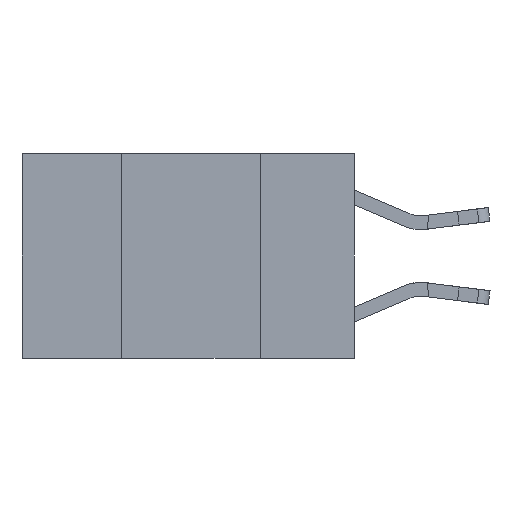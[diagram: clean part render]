
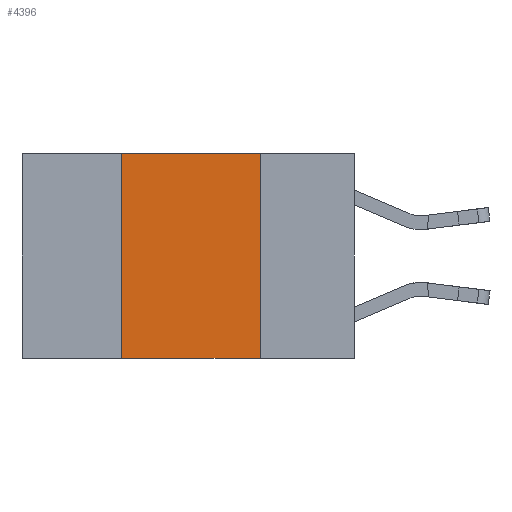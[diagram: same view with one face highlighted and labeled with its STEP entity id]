
A CAD part, left-side view. The second image highlights one B-rep face of the part: STEP entity #4396.
In plain terms, the highlighted planar face has unit normal (-1, 0, 0).
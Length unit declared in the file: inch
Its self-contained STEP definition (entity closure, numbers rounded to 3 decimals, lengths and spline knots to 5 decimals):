
#115 = CARTESIAN_POINT ( 'NONE',  ( 0., 0.42, 0. ) ) ;
#426 = VERTEX_POINT ( 'NONE', #19017 ) ;
#518 = LINE ( 'NONE', #115, #14392 ) ;
#2198 = CARTESIAN_POINT ( 'NONE',  ( 0., 0.42, -0.37 ) ) ;
#3190 = DIRECTION ( 'NONE',  ( 1., 0., 0. ) ) ;
#3238 = VECTOR ( 'NONE', #23253, 39.37008 ) ;
#3935 = ORIENTED_EDGE ( 'NONE', *, *, #14655, .F. ) ;
#4396 = ADVANCED_FACE ( 'NONE', ( #26177 ), #24254, .F. ) ;
#5618 = LINE ( 'NONE', #13851, #10953 ) ;
#5630 = CARTESIAN_POINT ( 'NONE',  ( 0., 0.17, 0. ) ) ;
#6776 = CARTESIAN_POINT ( 'NONE',  ( 0., 0.6, 0. ) ) ;
#6867 = VERTEX_POINT ( 'NONE', #2198 ) ;
#8411 = DIRECTION ( 'NONE',  ( 0., 0., 1. ) ) ;
#9534 = CARTESIAN_POINT ( 'NONE',  ( 0., 0.6, 0. ) ) ;
#9724 = VERTEX_POINT ( 'NONE', #19288 ) ;
#10010 = EDGE_CURVE ( 'NONE', #426, #16663, #16046, .T. ) ;
#10270 = AXIS2_PLACEMENT_3D ( 'NONE', #9534, #3190, #20065 ) ;
#10953 = VECTOR ( 'NONE', #21573, 39.37008 ) ;
#13851 = CARTESIAN_POINT ( 'NONE',  ( 0., 0.6, -0.37 ) ) ;
#13915 = EDGE_CURVE ( 'NONE', #6867, #16663, #5618, .T. ) ;
#14392 = VECTOR ( 'NONE', #8411, 39.37008 ) ;
#14655 = EDGE_CURVE ( 'NONE', #9724, #426, #14875, .T. ) ;
#14875 = LINE ( 'NONE', #6776, #3238 ) ;
#15882 = CARTESIAN_POINT ( 'NONE',  ( 0., 0.17, -0.37 ) ) ;
#16046 = LINE ( 'NONE', #5630, #24516 ) ;
#16663 = VERTEX_POINT ( 'NONE', #15882 ) ;
#17293 = EDGE_LOOP ( 'NONE', ( #22100, #3935, #23377, #23864 ) ) ;
#19017 = CARTESIAN_POINT ( 'NONE',  ( 0., 0.17, 0. ) ) ;
#19288 = CARTESIAN_POINT ( 'NONE',  ( 0., 0.42, 0. ) ) ;
#20065 = DIRECTION ( 'NONE',  ( 0., 0., -1. ) ) ;
#20082 = DIRECTION ( 'NONE',  ( 0., 0., -1. ) ) ;
#21573 = DIRECTION ( 'NONE',  ( 0., -1., 0. ) ) ;
#22100 = ORIENTED_EDGE ( 'NONE', *, *, #10010, .F. ) ;
#23253 = DIRECTION ( 'NONE',  ( 0., -1., 0. ) ) ;
#23377 = ORIENTED_EDGE ( 'NONE', *, *, #26283, .F. ) ;
#23864 = ORIENTED_EDGE ( 'NONE', *, *, #13915, .T. ) ;
#24254 = PLANE ( 'NONE',  #10270 ) ;
#24516 = VECTOR ( 'NONE', #20082, 39.37008 ) ;
#26177 = FACE_OUTER_BOUND ( 'NONE', #17293, .T. ) ;
#26283 = EDGE_CURVE ( 'NONE', #6867, #9724, #518, .T. ) ;
